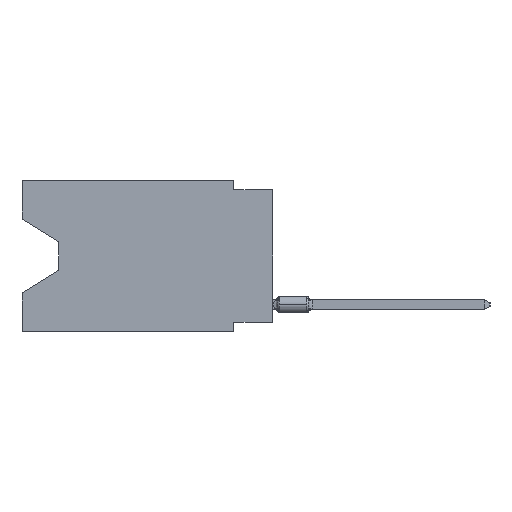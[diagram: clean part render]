
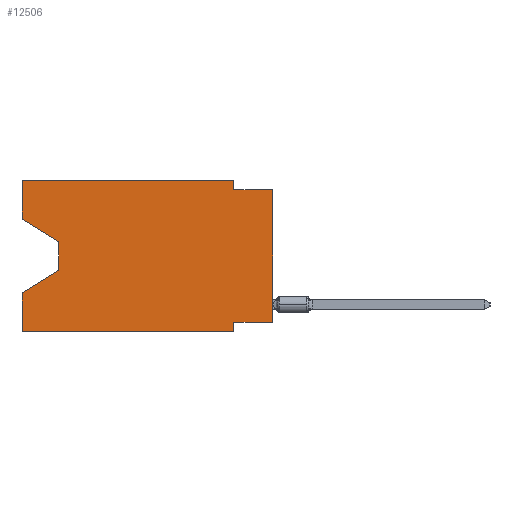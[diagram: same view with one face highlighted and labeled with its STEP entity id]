
A CAD part, left-side view. The second image highlights one B-rep face of the part: STEP entity #12506.
In plain terms, the highlighted planar face has unit normal (-1, 0, 0).
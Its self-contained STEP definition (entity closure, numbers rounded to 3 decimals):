
#346 = VECTOR ( 'NONE', #25639, 1000. ) ;
#561 = VECTOR ( 'NONE', #24291, 1000. ) ;
#579 = VECTOR ( 'NONE', #3349, 1000. ) ;
#850 = CARTESIAN_POINT ( 'NONE',  ( 0., 13.97, -5.893 ) ) ;
#1783 = DIRECTION ( 'NONE',  ( 0., 0., 1. ) ) ;
#2094 = CARTESIAN_POINT ( 'NONE',  ( 0., 2.54, -9.271 ) ) ;
#2313 = DIRECTION ( 'NONE',  ( 0., 0., -1. ) ) ;
#2406 = DIRECTION ( 'NONE',  ( 0., 0., -1. ) ) ;
#3186 = DIRECTION ( 'NONE',  ( 0., 0., 1. ) ) ;
#3346 = VECTOR ( 'NONE', #18513, 1000. ) ;
#3349 = DIRECTION ( 'NONE',  ( 0., 0., 1. ) ) ;
#4429 = VERTEX_POINT ( 'NONE', #39513 ) ;
#4686 = ORIENTED_EDGE ( 'NONE', *, *, #18288, .T. ) ;
#4728 = EDGE_CURVE ( 'NONE', #7957, #29069, #41378, .T. ) ;
#4943 = ORIENTED_EDGE ( 'NONE', *, *, #38479, .T. ) ;
#4987 = LINE ( 'NONE', #31285, #18380 ) ;
#5048 = VECTOR ( 'NONE', #19535, 1000. ) ;
#5055 = ORIENTED_EDGE ( 'NONE', *, *, #38964, .F. ) ;
#5434 = ORIENTED_EDGE ( 'NONE', *, *, #15884, .T. ) ;
#5604 = CARTESIAN_POINT ( 'NONE',  ( 0., 16.383, -7.36 ) ) ;
#5655 = LINE ( 'NONE', #41176, #3346 ) ;
#7951 = DIRECTION ( 'NONE',  ( 0., -0.855, -0.519 ) ) ;
#7957 = VERTEX_POINT ( 'NONE', #20346 ) ;
#8849 = DIRECTION ( 'NONE',  ( 0., 0., -1. ) ) ;
#8905 = LINE ( 'NONE', #21754, #561 ) ;
#9342 = CARTESIAN_POINT ( 'NONE',  ( 0., 2.54, -9.906 ) ) ;
#10652 = VERTEX_POINT ( 'NONE', #40383 ) ;
#11133 = VECTOR ( 'NONE', #2313, 1000. ) ;
#12008 = LINE ( 'NONE', #18540, #13077 ) ;
#12506 = ADVANCED_FACE ( 'NONE', ( #37335 ), #18421, .F. ) ;
#12620 = ORIENTED_EDGE ( 'NONE', *, *, #20246, .F. ) ;
#13077 = VECTOR ( 'NONE', #8849, 1000. ) ;
#13162 = VECTOR ( 'NONE', #18841, 1000. ) ;
#13283 = VERTEX_POINT ( 'NONE', #22197 ) ;
#14962 = CARTESIAN_POINT ( 'NONE',  ( 0., 2.54, 0. ) ) ;
#15360 = ORIENTED_EDGE ( 'NONE', *, *, #37522, .T. ) ;
#15570 = CARTESIAN_POINT ( 'NONE',  ( 0., 16.383, 0. ) ) ;
#15764 = CARTESIAN_POINT ( 'NONE',  ( 0., 16.383, -9.906 ) ) ;
#15884 = EDGE_CURVE ( 'NONE', #34443, #25435, #8905, .T. ) ;
#17577 = EDGE_CURVE ( 'NONE', #29069, #32802, #24856, .T. ) ;
#18288 = EDGE_CURVE ( 'NONE', #20624, #34443, #12008, .T. ) ;
#18380 = VECTOR ( 'NONE', #7951, 1000. ) ;
#18387 = CARTESIAN_POINT ( 'NONE',  ( 0., 0., -0.635 ) ) ;
#18420 = CARTESIAN_POINT ( 'NONE',  ( 0., 2.54, -0.635 ) ) ;
#18421 = PLANE ( 'NONE',  #23226 ) ;
#18513 = DIRECTION ( 'NONE',  ( 0., 1., 0. ) ) ;
#18540 = CARTESIAN_POINT ( 'NONE',  ( 0., 13.97, -4.013 ) ) ;
#18841 = DIRECTION ( 'NONE',  ( 0., -1., 0. ) ) ;
#19270 = ORIENTED_EDGE ( 'NONE', *, *, #4728, .F. ) ;
#19478 = EDGE_CURVE ( 'NONE', #13283, #4429, #22086, .T. ) ;
#19535 = DIRECTION ( 'NONE',  ( 0., -1., 0. ) ) ;
#20246 = EDGE_CURVE ( 'NONE', #40009, #4429, #38338, .T. ) ;
#20294 = VERTEX_POINT ( 'NONE', #18387 ) ;
#20346 = CARTESIAN_POINT ( 'NONE',  ( 0., 16.383, 0. ) ) ;
#20624 = VERTEX_POINT ( 'NONE', #28806 ) ;
#21262 = CARTESIAN_POINT ( 'NONE',  ( 0., 16.383, -2.546 ) ) ;
#21754 = CARTESIAN_POINT ( 'NONE',  ( 0., 13.97, -5.893 ) ) ;
#22086 = LINE ( 'NONE', #15764, #346 ) ;
#22197 = CARTESIAN_POINT ( 'NONE',  ( 0., 16.383, -9.906 ) ) ;
#23226 = AXIS2_PLACEMENT_3D ( 'NONE', #40470, #30625, #2406 ) ;
#24291 = DIRECTION ( 'NONE',  ( 0., 0.855, -0.519 ) ) ;
#24856 = LINE ( 'NONE', #14962, #11133 ) ;
#25082 = EDGE_CURVE ( 'NONE', #34529, #7957, #34901, .T. ) ;
#25435 = VERTEX_POINT ( 'NONE', #5604 ) ;
#25639 = DIRECTION ( 'NONE',  ( 0., -1., 0. ) ) ;
#27996 = VECTOR ( 'NONE', #1783, 1000. ) ;
#28806 = CARTESIAN_POINT ( 'NONE',  ( 0., 13.97, -4.013 ) ) ;
#28863 = CARTESIAN_POINT ( 'NONE',  ( 0., 0., 0. ) ) ;
#29006 = CARTESIAN_POINT ( 'NONE',  ( 0., 16.383, 0. ) ) ;
#29069 = VERTEX_POINT ( 'NONE', #31373 ) ;
#29131 = LINE ( 'NONE', #35426, #13162 ) ;
#29941 = ORIENTED_EDGE ( 'NONE', *, *, #19478, .T. ) ;
#29964 = VECTOR ( 'NONE', #35187, 1000. ) ;
#30155 = ORIENTED_EDGE ( 'NONE', *, *, #33816, .F. ) ;
#30610 = CARTESIAN_POINT ( 'NONE',  ( 0., 16.383, 0. ) ) ;
#30625 = DIRECTION ( 'NONE',  ( 1., 0., 0. ) ) ;
#31285 = CARTESIAN_POINT ( 'NONE',  ( 0., 16.383, -2.546 ) ) ;
#31373 = CARTESIAN_POINT ( 'NONE',  ( 0., 2.54, 0. ) ) ;
#31819 = ORIENTED_EDGE ( 'NONE', *, *, #32914, .F. ) ;
#32382 = ORIENTED_EDGE ( 'NONE', *, *, #25082, .F. ) ;
#32802 = VERTEX_POINT ( 'NONE', #18420 ) ;
#32914 = EDGE_CURVE ( 'NONE', #32802, #20294, #29131, .T. ) ;
#33139 = ORIENTED_EDGE ( 'NONE', *, *, #17577, .F. ) ;
#33741 = LINE ( 'NONE', #30610, #27996 ) ;
#33816 = EDGE_CURVE ( 'NONE', #13283, #25435, #33741, .T. ) ;
#34443 = VERTEX_POINT ( 'NONE', #850 ) ;
#34529 = VERTEX_POINT ( 'NONE', #21262 ) ;
#34901 = LINE ( 'NONE', #15570, #579 ) ;
#34947 = LINE ( 'NONE', #28863, #40896 ) ;
#35187 = DIRECTION ( 'NONE',  ( 0., 0., -1. ) ) ;
#35426 = CARTESIAN_POINT ( 'NONE',  ( 0., 0., -0.635 ) ) ;
#37335 = FACE_OUTER_BOUND ( 'NONE', #37599, .T. ) ;
#37522 = EDGE_CURVE ( 'NONE', #34529, #20624, #4987, .T. ) ;
#37599 = EDGE_LOOP ( 'NONE', ( #15360, #4686, #5434, #30155, #29941, #12620, #5055, #4943, #31819, #33139, #19270, #32382 ) ) ;
#38338 = LINE ( 'NONE', #9342, #29964 ) ;
#38479 = EDGE_CURVE ( 'NONE', #10652, #20294, #34947, .T. ) ;
#38964 = EDGE_CURVE ( 'NONE', #10652, #40009, #5655, .T. ) ;
#39513 = CARTESIAN_POINT ( 'NONE',  ( 0., 2.54, -9.906 ) ) ;
#40009 = VERTEX_POINT ( 'NONE', #2094 ) ;
#40383 = CARTESIAN_POINT ( 'NONE',  ( 0., 0., -9.271 ) ) ;
#40470 = CARTESIAN_POINT ( 'NONE',  ( 0., 16.383, 0. ) ) ;
#40896 = VECTOR ( 'NONE', #3186, 1000. ) ;
#41176 = CARTESIAN_POINT ( 'NONE',  ( 0., 0., -9.271 ) ) ;
#41378 = LINE ( 'NONE', #29006, #5048 ) ;
